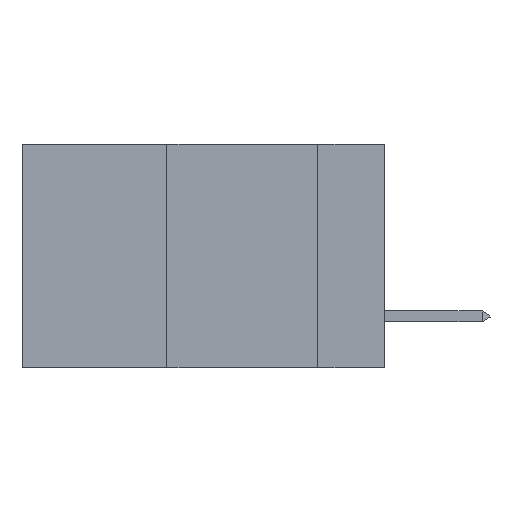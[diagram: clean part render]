
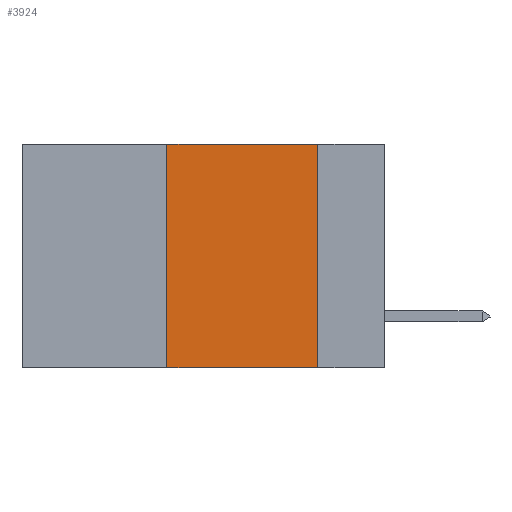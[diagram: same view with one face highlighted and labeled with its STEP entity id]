
A CAD part, left-side view. The second image highlights one B-rep face of the part: STEP entity #3924.
In plain terms, the highlighted planar face has unit normal (-1, 0, 0).
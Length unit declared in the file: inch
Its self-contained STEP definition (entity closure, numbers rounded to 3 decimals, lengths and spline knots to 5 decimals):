
#165 = LINE ( 'NONE', #15234, #16946 ) ;
#538 = DIRECTION ( 'NONE',  ( 0., 0., -1. ) ) ;
#929 = PLANE ( 'NONE',  #30586 ) ;
#1635 = LINE ( 'NONE', #15860, #31051 ) ;
#3924 = ADVANCED_FACE ( 'NONE', ( #32178 ), #929, .F. ) ;
#7196 = CARTESIAN_POINT ( 'NONE',  ( 0., 0.11, 0. ) ) ;
#9308 = EDGE_CURVE ( 'NONE', #33062, #12452, #22724, .T. ) ;
#10810 = CARTESIAN_POINT ( 'NONE',  ( 0., 0.11, -0.37 ) ) ;
#12374 = DIRECTION ( 'NONE',  ( 0., 0., 1. ) ) ;
#12452 = VERTEX_POINT ( 'NONE', #10810 ) ;
#14248 = VERTEX_POINT ( 'NONE', #18068 ) ;
#14269 = VECTOR ( 'NONE', #22192, 39.37008 ) ;
#15234 = CARTESIAN_POINT ( 'NONE',  ( 0., 0.6, -0.37 ) ) ;
#15648 = EDGE_CURVE ( 'NONE', #15734, #33062, #1635, .T. ) ;
#15734 = VERTEX_POINT ( 'NONE', #28141 ) ;
#15860 = CARTESIAN_POINT ( 'NONE',  ( 0., 0.6, 0. ) ) ;
#15991 = DIRECTION ( 'NONE',  ( 0., -1., 0. ) ) ;
#16581 = EDGE_LOOP ( 'NONE', ( #21333, #32124, #20390, #28308 ) ) ;
#16926 = VECTOR ( 'NONE', #12374, 39.37008 ) ;
#16946 = VECTOR ( 'NONE', #24381, 39.37008 ) ;
#18068 = CARTESIAN_POINT ( 'NONE',  ( 0., 0.36, -0.37 ) ) ;
#18627 = CARTESIAN_POINT ( 'NONE',  ( 0., 0.6, 0. ) ) ;
#18873 = DIRECTION ( 'NONE',  ( 1., 0., 0. ) ) ;
#20390 = ORIENTED_EDGE ( 'NONE', *, *, #34437, .F. ) ;
#21333 = ORIENTED_EDGE ( 'NONE', *, *, #9308, .F. ) ;
#22192 = DIRECTION ( 'NONE',  ( 0., 0., -1. ) ) ;
#22724 = LINE ( 'NONE', #7196, #14269 ) ;
#24244 = CARTESIAN_POINT ( 'NONE',  ( 0., 0.11, 0. ) ) ;
#24381 = DIRECTION ( 'NONE',  ( 0., -1., 0. ) ) ;
#24861 = EDGE_CURVE ( 'NONE', #14248, #12452, #165, .T. ) ;
#28141 = CARTESIAN_POINT ( 'NONE',  ( 0., 0.36, 0. ) ) ;
#28308 = ORIENTED_EDGE ( 'NONE', *, *, #24861, .T. ) ;
#30586 = AXIS2_PLACEMENT_3D ( 'NONE', #18627, #18873, #538 ) ;
#31051 = VECTOR ( 'NONE', #15991, 39.37008 ) ;
#32124 = ORIENTED_EDGE ( 'NONE', *, *, #15648, .F. ) ;
#32178 = FACE_OUTER_BOUND ( 'NONE', #16581, .T. ) ;
#33062 = VERTEX_POINT ( 'NONE', #24244 ) ;
#34437 = EDGE_CURVE ( 'NONE', #14248, #15734, #34705, .T. ) ;
#34705 = LINE ( 'NONE', #35917, #16926 ) ;
#35917 = CARTESIAN_POINT ( 'NONE',  ( 0., 0.36, 0. ) ) ;
